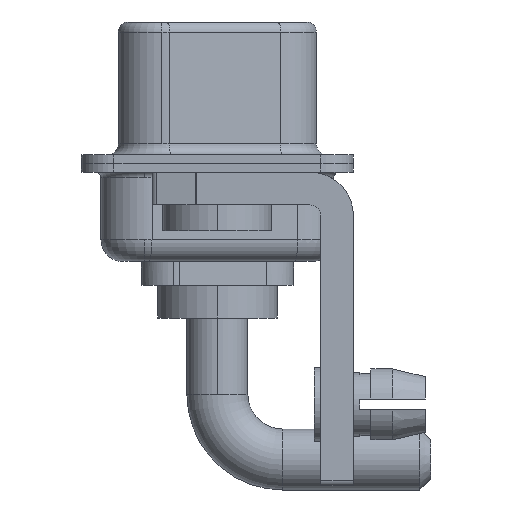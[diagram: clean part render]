
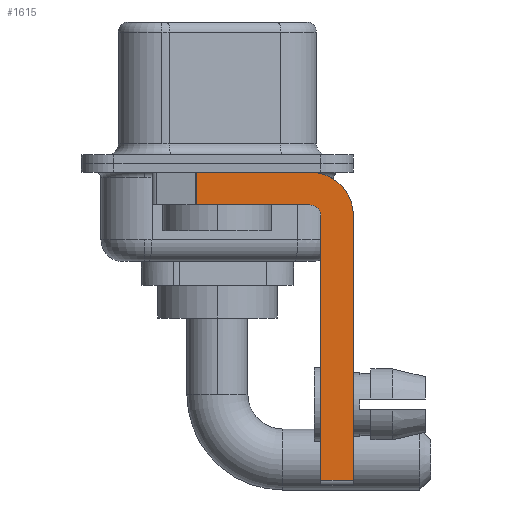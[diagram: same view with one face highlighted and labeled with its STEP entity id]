
A CAD part, left-side view. The second image highlights one B-rep face of the part: STEP entity #1615.
In plain terms, the highlighted planar face has unit normal (-1, 0, 0).
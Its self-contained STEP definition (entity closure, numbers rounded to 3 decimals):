
#582 = AXIS2_PLACEMENT_3D ( 'NONE', #841, #3522, #8727 ) ;
#720 = EDGE_CURVE ( 'NONE', #1066, #10190, #1920, .T. ) ;
#841 = CARTESIAN_POINT ( 'NONE',  ( -2.9, -4.25, -2.4 ) ) ;
#951 = CARTESIAN_POINT ( 'NONE',  ( -2.9, 0.978, -1.9 ) ) ;
#952 = DIRECTION ( 'NONE',  ( 0., 1., 0. ) ) ;
#1050 = DIRECTION ( 'NONE',  ( 1., 0., 0. ) ) ;
#1066 = VERTEX_POINT ( 'NONE', #4063 ) ;
#1615 = ADVANCED_FACE ( 'NONE', ( #5076 ), #13032, .F. ) ;
#1920 = LINE ( 'NONE', #6821, #4817 ) ;
#2028 = CARTESIAN_POINT ( 'NONE',  ( -2.9, 3., -0.4 ) ) ;
#2408 = CARTESIAN_POINT ( 'NONE',  ( -2.9, -6.25, -2.4 ) ) ;
#2437 = VERTEX_POINT ( 'NONE', #5199 ) ;
#2487 = DIRECTION ( 'NONE',  ( 0., 0., -1. ) ) ;
#2653 = EDGE_CURVE ( 'NONE', #6857, #16733, #8584, .T. ) ;
#2668 = ORIENTED_EDGE ( 'NONE', *, *, #12099, .F. ) ;
#2762 = ORIENTED_EDGE ( 'NONE', *, *, #16408, .F. ) ;
#2825 = ORIENTED_EDGE ( 'NONE', *, *, #11006, .F. ) ;
#2895 = ORIENTED_EDGE ( 'NONE', *, *, #15401, .F. ) ;
#3242 = DIRECTION ( 'NONE',  ( 0., -1., 0. ) ) ;
#3243 = VECTOR ( 'NONE', #3242, 1000. ) ;
#3522 = DIRECTION ( 'NONE',  ( -1., 0., 0. ) ) ;
#3966 = CARTESIAN_POINT ( 'NONE',  ( -2.9, -6.25, -14.55 ) ) ;
#4063 = CARTESIAN_POINT ( 'NONE',  ( -2.9, -4.75, -14.55 ) ) ;
#4515 = EDGE_CURVE ( 'NONE', #1066, #8591, #11896, .T. ) ;
#4817 = VECTOR ( 'NONE', #7078, 1000. ) ;
#4933 = CARTESIAN_POINT ( 'NONE',  ( -2.9, -4.25, -2.4 ) ) ;
#5076 = FACE_OUTER_BOUND ( 'NONE', #13809, .T. ) ;
#5199 = CARTESIAN_POINT ( 'NONE',  ( -2.9, -4.25, -1.9 ) ) ;
#5265 = CARTESIAN_POINT ( 'NONE',  ( -2.9, 0.978, -0.4 ) ) ;
#6690 = AXIS2_PLACEMENT_3D ( 'NONE', #4933, #1050, #16743 ) ;
#6821 = CARTESIAN_POINT ( 'NONE',  ( -2.9, -4.75, -14.8 ) ) ;
#6857 = VERTEX_POINT ( 'NONE', #5265 ) ;
#7078 = DIRECTION ( 'NONE',  ( 0., 0., 1. ) ) ;
#7872 = DIRECTION ( 'NONE',  ( 0., -1., 0. ) ) ;
#8188 = CARTESIAN_POINT ( 'NONE',  ( -2.9, -4.25, -1.9 ) ) ;
#8193 = ORIENTED_EDGE ( 'NONE', *, *, #720, .F. ) ;
#8584 = LINE ( 'NONE', #951, #16665 ) ;
#8591 = VERTEX_POINT ( 'NONE', #3966 ) ;
#8616 = VECTOR ( 'NONE', #13444, 1000. ) ;
#8727 = DIRECTION ( 'NONE',  ( 0., 0., 1. ) ) ;
#8991 = CARTESIAN_POINT ( 'NONE',  ( -2.9, -4.25, -2.4 ) ) ;
#9825 = LINE ( 'NONE', #2028, #3243 ) ;
#9828 = VECTOR ( 'NONE', #7872, 1000. ) ;
#10190 = VERTEX_POINT ( 'NONE', #10762 ) ;
#10288 = DIRECTION ( 'NONE',  ( 1., 0., 0. ) ) ;
#10762 = CARTESIAN_POINT ( 'NONE',  ( -2.9, -4.75, -2.4 ) ) ;
#11006 = EDGE_CURVE ( 'NONE', #12921, #16007, #15994, .T. ) ;
#11052 = ORIENTED_EDGE ( 'NONE', *, *, #2653, .T. ) ;
#11500 = AXIS2_PLACEMENT_3D ( 'NONE', #8991, #10288, #2487 ) ;
#11553 = CARTESIAN_POINT ( 'NONE',  ( -2.9, -4.25, -14.55 ) ) ;
#11831 = CIRCLE ( 'NONE', #582, 0.5 ) ;
#11896 = LINE ( 'NONE', #11553, #9828 ) ;
#12099 = EDGE_CURVE ( 'NONE', #16007, #8591, #13192, .T. ) ;
#12521 = VECTOR ( 'NONE', #952, 1000. ) ;
#12853 = CARTESIAN_POINT ( 'NONE',  ( -2.9, -6.25, -2.4 ) ) ;
#12921 = VERTEX_POINT ( 'NONE', #15788 ) ;
#13032 = PLANE ( 'NONE',  #11500 ) ;
#13192 = LINE ( 'NONE', #12853, #8616 ) ;
#13308 = ORIENTED_EDGE ( 'NONE', *, *, #15882, .F. ) ;
#13444 = DIRECTION ( 'NONE',  ( 0., 0., -1. ) ) ;
#13809 = EDGE_LOOP ( 'NONE', ( #2895, #11052, #13308, #2762, #8193, #13918, #2668, #2825 ) ) ;
#13918 = ORIENTED_EDGE ( 'NONE', *, *, #4515, .T. ) ;
#13987 = DIRECTION ( 'NONE',  ( 0., 0., -1. ) ) ;
#14391 = CARTESIAN_POINT ( 'NONE',  ( -2.9, 0.978, -1.9 ) ) ;
#15401 = EDGE_CURVE ( 'NONE', #6857, #12921, #9825, .T. ) ;
#15788 = CARTESIAN_POINT ( 'NONE',  ( -2.9, -4.25, -0.4 ) ) ;
#15882 = EDGE_CURVE ( 'NONE', #2437, #16733, #16078, .T. ) ;
#15994 = CIRCLE ( 'NONE', #6690, 2. ) ;
#16007 = VERTEX_POINT ( 'NONE', #2408 ) ;
#16078 = LINE ( 'NONE', #8188, #12521 ) ;
#16408 = EDGE_CURVE ( 'NONE', #10190, #2437, #11831, .T. ) ;
#16665 = VECTOR ( 'NONE', #13987, 1000. ) ;
#16733 = VERTEX_POINT ( 'NONE', #14391 ) ;
#16743 = DIRECTION ( 'NONE',  ( 0., 0., -1. ) ) ;
